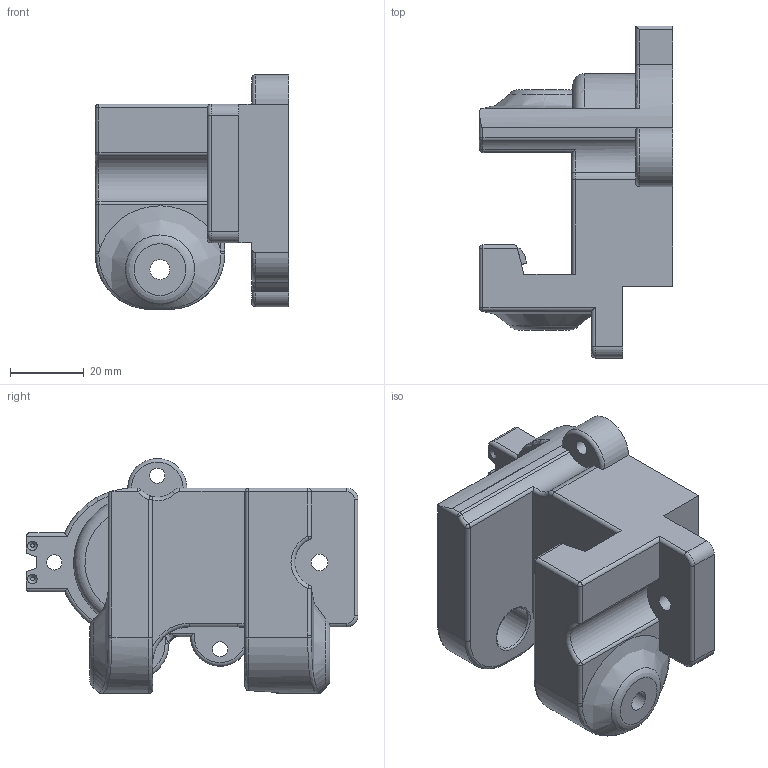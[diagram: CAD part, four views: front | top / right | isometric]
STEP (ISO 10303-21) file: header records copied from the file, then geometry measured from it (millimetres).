
FILE_DESCRIPTION (( 'STEP AP203' ), '1' );
FILE_NAME ('WTF-9_rear_end_cap.STEP', '2020-05-09T09:29:57', ( '' ), ( '' ), 'SwSTEP 2.0', 'SolidWorks 2016', '' );
FILE_SCHEMA (( 'CONFIG_CONTROL_DESIGN' ));
Length unit declared in the file: millimetre
Products named in the file (2): WTF-9_rear_end_cap; WTF9 V1 FINAL_6
Assembly tree (1 placements, depth 2):
  WTF-9_rear_end_cap
    WTF9 V1 FINAL_6
Bounding box: 52.33 x 89.8 x 63.54 mm (x, y, z)
Volume: 99808.5 mm3; surface area: 24195.7 mm2
Topology: 1 solids, 1 shells, 180 faces, 448 edges, 270 vertices
Faces by surface type: cylinder 68, plane 53, torus 27, bspline 17, cone 8, sphere 7
Full cylindrical faces by diameter (mm): 1 x2, 4.1 x3, 4.5 x1, 5.4 x2, 12 x1, 22 x1
Entity records: 7021 total; most frequent: CARTESIAN_POINT 2829, ORIENTED_EDGE 832, DIRECTION 800, EDGE_CURVE 416, AXIS2_PLACEMENT_3D 313, VERTEX_POINT 266, EDGE_LOOP 220, FACE_OUTER_BOUND 195
